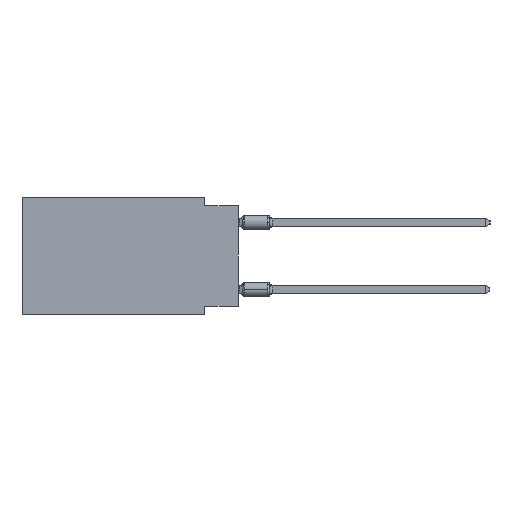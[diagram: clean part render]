
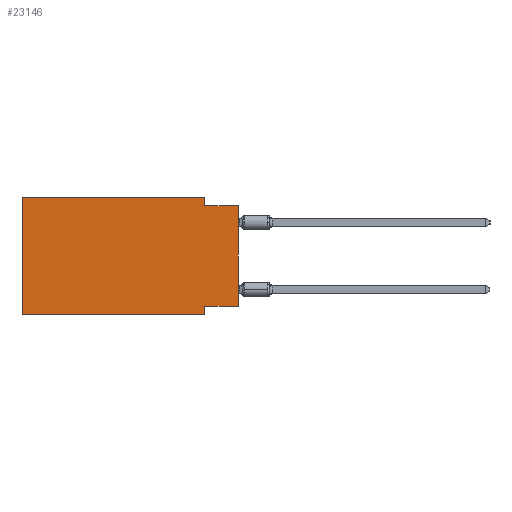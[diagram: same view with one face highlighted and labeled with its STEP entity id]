
A CAD part, left-side view. The second image highlights one B-rep face of the part: STEP entity #23146.
In plain terms, the highlighted planar face has unit normal (-1, 0, 0).
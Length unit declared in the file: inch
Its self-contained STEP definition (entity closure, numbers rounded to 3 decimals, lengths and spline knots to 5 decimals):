
#767 = EDGE_LOOP ( 'NONE', ( #1371, #29825, #8093, #20470, #12480, #14409, #29634, #12954 ) ) ;
#1112 = PLANE ( 'NONE',  #2014 ) ;
#1125 = LINE ( 'NONE', #27321, #20391 ) ;
#1371 = ORIENTED_EDGE ( 'NONE', *, *, #7726, .T. ) ;
#1539 = VERTEX_POINT ( 'NONE', #19041 ) ;
#1961 = CARTESIAN_POINT ( 'NONE',  ( 0., 0.1, 0. ) ) ;
#2014 = AXIS2_PLACEMENT_3D ( 'NONE', #24484, #14753, #10646 ) ;
#2087 = EDGE_CURVE ( 'NONE', #4999, #21252, #6694, .T. ) ;
#2376 = LINE ( 'NONE', #9713, #15496 ) ;
#2452 = VECTOR ( 'NONE', #13890, 39.37008 ) ;
#2695 = CARTESIAN_POINT ( 'NONE',  ( 0., 0.1, -0.025 ) ) ;
#3763 = DIRECTION ( 'NONE',  ( 0., 0., 1. ) ) ;
#3796 = DIRECTION ( 'NONE',  ( 0., 0., -1. ) ) ;
#4563 = DIRECTION ( 'NONE',  ( 0., 0., -1. ) ) ;
#4763 = CARTESIAN_POINT ( 'NONE',  ( 0., 0.645, -0.35 ) ) ;
#4852 = VERTEX_POINT ( 'NONE', #1961 ) ;
#4999 = VERTEX_POINT ( 'NONE', #2695 ) ;
#5960 = CARTESIAN_POINT ( 'NONE',  ( 0., 0.645, 0. ) ) ;
#6694 = LINE ( 'NONE', #16280, #11502 ) ;
#6978 = VECTOR ( 'NONE', #3763, 39.37008 ) ;
#7726 = EDGE_CURVE ( 'NONE', #21678, #21252, #14073, .T. ) ;
#8093 = ORIENTED_EDGE ( 'NONE', *, *, #22933, .F. ) ;
#8299 = VECTOR ( 'NONE', #3796, 39.37008 ) ;
#8434 = EDGE_CURVE ( 'NONE', #12776, #23757, #17021, .T. ) ;
#9496 = DIRECTION ( 'NONE',  ( 0., -1., 0. ) ) ;
#9713 = CARTESIAN_POINT ( 'NONE',  ( 0., 0.1, 0. ) ) ;
#10646 = DIRECTION ( 'NONE',  ( 0., 0., -1. ) ) ;
#11319 = LINE ( 'NONE', #27501, #8299 ) ;
#11502 = VECTOR ( 'NONE', #9496, 39.37008 ) ;
#12480 = ORIENTED_EDGE ( 'NONE', *, *, #23373, .F. ) ;
#12776 = VERTEX_POINT ( 'NONE', #19215 ) ;
#12954 = ORIENTED_EDGE ( 'NONE', *, *, #13893, .F. ) ;
#13890 = DIRECTION ( 'NONE',  ( 0., -1., 0. ) ) ;
#13893 = EDGE_CURVE ( 'NONE', #21678, #1539, #1125, .T. ) ;
#14073 = LINE ( 'NONE', #14353, #27807 ) ;
#14353 = CARTESIAN_POINT ( 'NONE',  ( 0., 0., 0. ) ) ;
#14409 = ORIENTED_EDGE ( 'NONE', *, *, #8434, .T. ) ;
#14753 = DIRECTION ( 'NONE',  ( 1., 0., 0. ) ) ;
#15496 = VECTOR ( 'NONE', #4563, 39.37008 ) ;
#16280 = CARTESIAN_POINT ( 'NONE',  ( 0., 0., -0.025 ) ) ;
#17021 = LINE ( 'NONE', #4763, #25729 ) ;
#17041 = CARTESIAN_POINT ( 'NONE',  ( 0., 0.645, 0. ) ) ;
#17433 = FACE_OUTER_BOUND ( 'NONE', #767, .T. ) ;
#17509 = VERTEX_POINT ( 'NONE', #17041 ) ;
#17849 = LINE ( 'NONE', #18605, #2452 ) ;
#18605 = CARTESIAN_POINT ( 'NONE',  ( 0., 0.645, 0. ) ) ;
#19041 = CARTESIAN_POINT ( 'NONE',  ( 0., 0.1, -0.325 ) ) ;
#19215 = CARTESIAN_POINT ( 'NONE',  ( 0., 0.645, -0.35 ) ) ;
#19940 = DIRECTION ( 'NONE',  ( 0., 1., 0. ) ) ;
#20391 = VECTOR ( 'NONE', #19940, 39.37008 ) ;
#20470 = ORIENTED_EDGE ( 'NONE', *, *, #22375, .F. ) ;
#21252 = VERTEX_POINT ( 'NONE', #28097 ) ;
#21678 = VERTEX_POINT ( 'NONE', #25476 ) ;
#21727 = DIRECTION ( 'NONE',  ( 0., -1., 0. ) ) ;
#22375 = EDGE_CURVE ( 'NONE', #17509, #4852, #17849, .T. ) ;
#22933 = EDGE_CURVE ( 'NONE', #4852, #4999, #2376, .T. ) ;
#23146 = ADVANCED_FACE ( 'NONE', ( #17433 ), #1112, .F. ) ;
#23373 = EDGE_CURVE ( 'NONE', #12776, #17509, #25283, .T. ) ;
#23639 = DIRECTION ( 'NONE',  ( 0., 0., 1. ) ) ;
#23757 = VERTEX_POINT ( 'NONE', #30120 ) ;
#24484 = CARTESIAN_POINT ( 'NONE',  ( 0., 0.645, 0. ) ) ;
#25283 = LINE ( 'NONE', #5960, #6978 ) ;
#25476 = CARTESIAN_POINT ( 'NONE',  ( 0., 0., -0.325 ) ) ;
#25729 = VECTOR ( 'NONE', #21727, 39.37008 ) ;
#27321 = CARTESIAN_POINT ( 'NONE',  ( 0., 0., -0.325 ) ) ;
#27501 = CARTESIAN_POINT ( 'NONE',  ( 0., 0.1, -0.35 ) ) ;
#27807 = VECTOR ( 'NONE', #23639, 39.37008 ) ;
#28097 = CARTESIAN_POINT ( 'NONE',  ( 0., 0., -0.025 ) ) ;
#29634 = ORIENTED_EDGE ( 'NONE', *, *, #30241, .F. ) ;
#29825 = ORIENTED_EDGE ( 'NONE', *, *, #2087, .F. ) ;
#30120 = CARTESIAN_POINT ( 'NONE',  ( 0., 0.1, -0.35 ) ) ;
#30241 = EDGE_CURVE ( 'NONE', #1539, #23757, #11319, .T. ) ;
